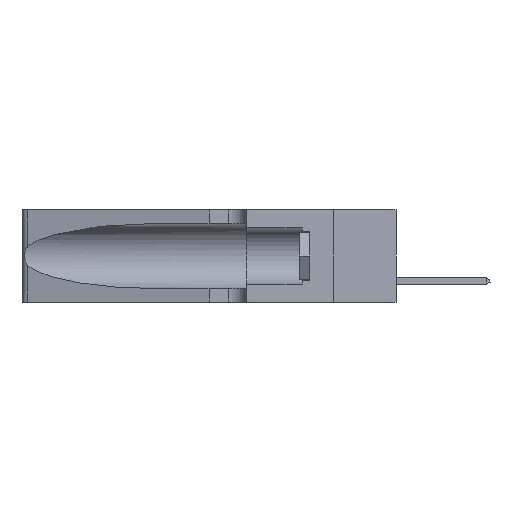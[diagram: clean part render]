
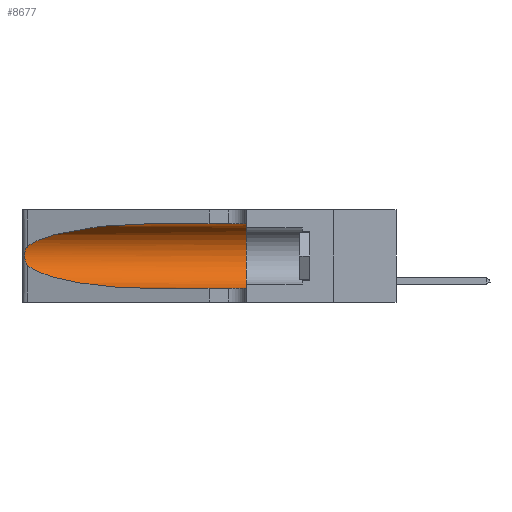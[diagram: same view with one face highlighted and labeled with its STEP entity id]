
A CAD part, left-side view. The second image highlights one B-rep face of the part: STEP entity #8677.
In plain terms, the highlighted cylindrical face has radius 3.308 mm (diameter 6.617 mm), a partial arc.
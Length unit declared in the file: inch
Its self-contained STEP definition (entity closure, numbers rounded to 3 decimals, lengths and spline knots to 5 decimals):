
#617 = CARTESIAN_POINT ( 'NONE',  ( 0.25639, 1.23186, 0.15144 ) ) ;
#805 = DIRECTION ( 'NONE',  ( 0., 1., 0. ) ) ;
#1795 = VERTEX_POINT ( 'NONE', #5998 ) ;
#2121 = DIRECTION ( 'NONE',  ( 0., -1., 0. ) ) ;
#2992 = CARTESIAN_POINT ( 'NONE',  ( 0.26075, 1.23896, 0.19203 ) ) ;
#3622 = EDGE_CURVE ( 'NONE', #10661, #29826, #20187, .T. ) ;
#4840 = CARTESIAN_POINT ( 'NONE',  ( 0.1305, 1.61858, 0.185 ) ) ;
#5830 = CARTESIAN_POINT ( 'NONE',  ( 0.18966, 0.96281, 0.05475 ) ) ;
#5998 = CARTESIAN_POINT ( 'NONE',  ( 0.1305, 0.35, 0.05475 ) ) ;
#6582 = CARTESIAN_POINT ( 'NONE',  ( 0.1305, 0.72297, 0.31525 ) ) ;
#7013 = ORIENTED_EDGE ( 'NONE', *, *, #3622, .T. ) ;
#7040 = CARTESIAN_POINT ( 'NONE',  ( 0.25487, 1.22718, 0.22369 ) ) ;
#7271 = ORIENTED_EDGE ( 'NONE', *, *, #9794, .T. ) ;
#7614 = EDGE_CURVE ( 'NONE', #16614, #1795, #15962, .T. ) ;
#8196 = CARTESIAN_POINT ( 'NONE',  ( 0.1305, 0.72297, 0.31525 ) ) ;
#8465 = CYLINDRICAL_SURFACE ( 'NONE', #25690, 0.13025 ) ;
#8677 = ADVANCED_FACE ( 'NONE', ( #8857 ), #8465, .F. ) ;
#8857 = FACE_OUTER_BOUND ( 'NONE', #21331, .T. ) ;
#8990 = CARTESIAN_POINT ( 'NONE',  ( 0.2373, 1.15595, 0.28018 ) ) ;
#9180 =( BOUNDED_CURVE ( )  B_SPLINE_CURVE ( 3, ( #6582, #28047, #8990, #18402 ),
 .UNSPECIFIED., .F., .T. ) 
 B_SPLINE_CURVE_WITH_KNOTS ( ( 4, 4 ),
 ( 1.5708, 2.84003 ),
 .UNSPECIFIED. ) 
 CURVE ( )  GEOMETRIC_REPRESENTATION_ITEM ( )  RATIONAL_B_SPLINE_CURVE ( ( 1., 0.87, 0.87, 1. ) ) 
 REPRESENTATION_ITEM ( '' )  );
#9794 = EDGE_CURVE ( 'NONE', #26977, #27611, #9180, .T. ) ;
#9969 = CARTESIAN_POINT ( 'NONE',  ( 0.2373, 1.15595, 0.08982 ) ) ;
#10661 = VERTEX_POINT ( 'NONE', #21464 ) ;
#11082 = CARTESIAN_POINT ( 'NONE',  ( 0.1305, 0.72297, 0.05475 ) ) ;
#11576 = AXIS2_PLACEMENT_3D ( 'NONE', #26921, #805, #21912 ) ;
#13643 = ORIENTED_EDGE ( 'NONE', *, *, #23845, .T. ) ;
#13666 = VECTOR ( 'NONE', #21655, 39.37008 ) ;
#13838 = EDGE_CURVE ( 'NONE', #26977, #16614, #18477, .T. ) ;
#14870 = CARTESIAN_POINT ( 'NONE',  ( 0.25854, 1.2359, 0.20912 ) ) ;
#14902 = CARTESIAN_POINT ( 'NONE',  ( 0.26017, 1.23833, 0.17102 ) ) ;
#15127 = CARTESIAN_POINT ( 'NONE',  ( 0.25487, 1.22718, 0.14631 ) ) ;
#15569 = CARTESIAN_POINT ( 'NONE',  ( 0.1305, 0.35, 0.31525 ) ) ;
#15962 = CIRCLE ( 'NONE', #11576, 0.13025 ) ;
#16225 = CARTESIAN_POINT ( 'NONE',  ( 0.26018, 1.23835, 0.19895 ) ) ;
#16614 = VERTEX_POINT ( 'NONE', #15569 ) ;
#16888 = CARTESIAN_POINT ( 'NONE',  ( 0.25487, 1.22718, 0.14631 ) ) ;
#17157 = VECTOR ( 'NONE', #2121, 39.37008 ) ;
#17271 = CARTESIAN_POINT ( 'NONE',  ( 0.25789, 1.23486, 0.15765 ) ) ;
#17707 = CARTESIAN_POINT ( 'NONE',  ( 0.25555, 1.22994, 0.2215 ) ) ;
#18402 = CARTESIAN_POINT ( 'NONE',  ( 0.25487, 1.22718, 0.22369 ) ) ;
#18477 = LINE ( 'NONE', #23827, #13666 ) ;
#19581 = CARTESIAN_POINT ( 'NONE',  ( 0.25555, 1.22993, 0.14849 ) ) ;
#19908 = CARTESIAN_POINT ( 'NONE',  ( 0.26075, 1.23896, 0.178 ) ) ;
#20187 =( BOUNDED_CURVE ( )  B_SPLINE_CURVE ( 3, ( #16888, #9969, #5830, #29557 ),
 .UNSPECIFIED., .F., .T. ) 
 B_SPLINE_CURVE_WITH_KNOTS ( ( 4, 4 ),
 ( 3.44316, 4.71239 ),
 .UNSPECIFIED. ) 
 CURVE ( )  GEOMETRIC_REPRESENTATION_ITEM ( )  RATIONAL_B_SPLINE_CURVE ( ( 1., 0.87, 0.87, 1. ) ) 
 REPRESENTATION_ITEM ( '' )  );
#21331 = EDGE_LOOP ( 'NONE', ( #7271, #13643, #7013, #21537, #27899, #26095 ) ) ;
#21464 = CARTESIAN_POINT ( 'NONE',  ( 0.25487, 1.22718, 0.14631 ) ) ;
#21537 = ORIENTED_EDGE ( 'NONE', *, *, #25929, .T. ) ;
#21655 = DIRECTION ( 'NONE',  ( 0., -1., 0. ) ) ;
#21912 = DIRECTION ( 'NONE',  ( 0., 0., 1. ) ) ;
#21922 = CARTESIAN_POINT ( 'NONE',  ( 0.25787, 1.23484, 0.2124 ) ) ;
#23827 = CARTESIAN_POINT ( 'NONE',  ( 0.1305, 1.61858, 0.31525 ) ) ;
#23845 = EDGE_CURVE ( 'NONE', #27611, #10661, #27424, .T. ) ;
#24853 = DIRECTION ( 'NONE',  ( 0., 0., -1. ) ) ;
#25175 = DIRECTION ( 'NONE',  ( 0., -1., 0. ) ) ;
#25346 = LINE ( 'NONE', #30525, #17157 ) ;
#25690 = AXIS2_PLACEMENT_3D ( 'NONE', #4840, #25175, #24853 ) ;
#25929 = EDGE_CURVE ( 'NONE', #29826, #1795, #25346, .T. ) ;
#26095 = ORIENTED_EDGE ( 'NONE', *, *, #13838, .F. ) ;
#26585 = CARTESIAN_POINT ( 'NONE',  ( 0.25639, 1.23184, 0.21858 ) ) ;
#26849 = CARTESIAN_POINT ( 'NONE',  ( 0.25856, 1.23593, 0.16098 ) ) ;
#26921 = CARTESIAN_POINT ( 'NONE',  ( 0.1305, 0.35, 0.185 ) ) ;
#26977 = VERTEX_POINT ( 'NONE', #8196 ) ;
#27424 = B_SPLINE_CURVE_WITH_KNOTS ( 'NONE', 3,
 ( #7040, #17707, #26585, #21922, #14870, #16225, #2992, #19908, #14902, #26849, #17271, #617, #19581, #15127 ),
 .UNSPECIFIED., .F., .F.,
 ( 4, 2, 2, 2, 2, 2, 4 ),
 ( 0., 0.00027, 0.00053, 0.00107, 0.0016, 0.00187, 0.00214 ),
 .UNSPECIFIED. ) ;
#27558 = CARTESIAN_POINT ( 'NONE',  ( 0.25487, 1.22718, 0.22369 ) ) ;
#27611 = VERTEX_POINT ( 'NONE', #27558 ) ;
#27899 = ORIENTED_EDGE ( 'NONE', *, *, #7614, .F. ) ;
#28047 = CARTESIAN_POINT ( 'NONE',  ( 0.18966, 0.96281, 0.31525 ) ) ;
#29557 = CARTESIAN_POINT ( 'NONE',  ( 0.1305, 0.72297, 0.05475 ) ) ;
#29826 = VERTEX_POINT ( 'NONE', #11082 ) ;
#30525 = CARTESIAN_POINT ( 'NONE',  ( 0.1305, 1.61858, 0.05475 ) ) ;
